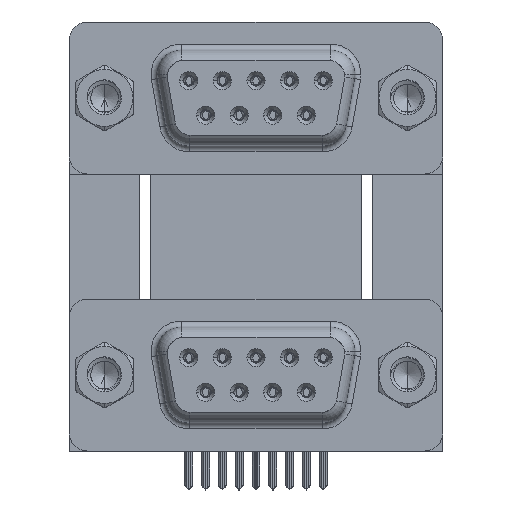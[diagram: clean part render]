
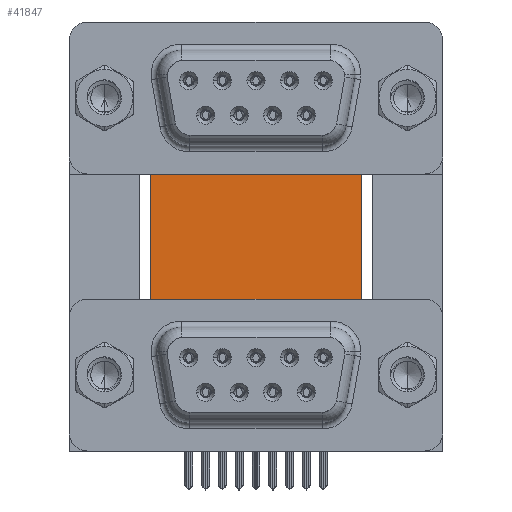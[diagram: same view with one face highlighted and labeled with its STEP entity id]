
A CAD part, top view. The second image highlights one B-rep face of the part: STEP entity #41847.
In plain terms, the highlighted planar face has unit normal (0, 0, 1).
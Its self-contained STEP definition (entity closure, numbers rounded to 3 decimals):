
#143 = EDGE_CURVE ( 'NONE', #31300, #3203, #23245, .T. ) ;
#572 = LINE ( 'NONE', #11947, #24037 ) ;
#943 = DIRECTION ( 'NONE',  ( -0.336, -0.942, 0. ) ) ;
#944 = LINE ( 'NONE', #15397, #3514 ) ;
#1466 = EDGE_CURVE ( 'NONE', #10846, #35164, #11918, .T. ) ;
#1846 = CARTESIAN_POINT ( 'NONE',  ( 3.79, 16.585, -12. ) ) ;
#2363 = VERTEX_POINT ( 'NONE', #5298 ) ;
#2872 = DIRECTION ( 'NONE',  ( 0., -1., 0. ) ) ;
#3203 = VERTEX_POINT ( 'NONE', #42561 ) ;
#3514 = VECTOR ( 'NONE', #33611, 1000. ) ;
#5298 = CARTESIAN_POINT ( 'NONE',  ( 3.79, 16.585, -12. ) ) ;
#5550 = LINE ( 'NONE', #23525, #19580 ) ;
#5804 = EDGE_CURVE ( 'NONE', #2363, #32591, #39345, .T. ) ;
#5820 = CARTESIAN_POINT ( 'NONE',  ( 22.59, -4.635, -12. ) ) ;
#6015 = EDGE_CURVE ( 'NONE', #22601, #10846, #944, .T. ) ;
#6263 = CARTESIAN_POINT ( 'NONE',  ( 2.9, -3.735, -12. ) ) ;
#6420 = ORIENTED_EDGE ( 'NONE', *, *, #22194, .T. ) ;
#8734 = FACE_OUTER_BOUND ( 'NONE', #43649, .T. ) ;
#10047 = VECTOR ( 'NONE', #26357, 1000. ) ;
#10072 = LINE ( 'NONE', #45401, #39113 ) ;
#10383 = DIRECTION ( 'NONE',  ( -0.336, 0.942, 0. ) ) ;
#10444 = VERTEX_POINT ( 'NONE', #33880 ) ;
#10846 = VERTEX_POINT ( 'NONE', #30279 ) ;
#11463 = LINE ( 'NONE', #18355, #26420 ) ;
#11918 = LINE ( 'NONE', #21882, #10047 ) ;
#11947 = CARTESIAN_POINT ( 'NONE',  ( 22.59, -4.635, -12. ) ) ;
#12884 = ORIENTED_EDGE ( 'NONE', *, *, #24307, .T. ) ;
#13352 = VERTEX_POINT ( 'NONE', #44751 ) ;
#13515 = VECTOR ( 'NONE', #943, 1000. ) ;
#13616 = EDGE_CURVE ( 'NONE', #2363, #31300, #21714, .T. ) ;
#13801 = VECTOR ( 'NONE', #21245, 1000. ) ;
#13911 = VERTEX_POINT ( 'NONE', #5820 ) ;
#13927 = ORIENTED_EDGE ( 'NONE', *, *, #6015, .T. ) ;
#15397 = CARTESIAN_POINT ( 'NONE',  ( 3.79, -3.735, -12. ) ) ;
#16994 = ORIENTED_EDGE ( 'NONE', *, *, #41532, .T. ) ;
#17718 = ORIENTED_EDGE ( 'NONE', *, *, #1466, .T. ) ;
#18168 = CARTESIAN_POINT ( 'NONE',  ( 21.2, 16.585, -12. ) ) ;
#18355 = CARTESIAN_POINT ( 'NONE',  ( 22.09, -4.635, -12. ) ) ;
#18534 = DIRECTION ( 'NONE',  ( 0., 0., -1. ) ) ;
#18956 = CARTESIAN_POINT ( 'NONE',  ( 2.4, -4.635, -12. ) ) ;
#19362 = ORIENTED_EDGE ( 'NONE', *, *, #37364, .T. ) ;
#19580 = VECTOR ( 'NONE', #20441, 1000. ) ;
#20441 = DIRECTION ( 'NONE',  ( 0., 1., 0. ) ) ;
#21245 = DIRECTION ( 'NONE',  ( 1., 0., 0. ) ) ;
#21714 = LINE ( 'NONE', #42338, #13801 ) ;
#21882 = CARTESIAN_POINT ( 'NONE',  ( 22.09, -3.735, -12. ) ) ;
#22131 = DIRECTION ( 'NONE',  ( 1., 0., 0. ) ) ;
#22194 = EDGE_CURVE ( 'NONE', #10444, #13352, #10072, .T. ) ;
#22601 = VERTEX_POINT ( 'NONE', #6263 ) ;
#23245 = LINE ( 'NONE', #30788, #34875 ) ;
#23525 = CARTESIAN_POINT ( 'NONE',  ( 2.9, -3.735, -12. ) ) ;
#24037 = VECTOR ( 'NONE', #10383, 1000. ) ;
#24307 = EDGE_CURVE ( 'NONE', #32591, #10444, #40762, .T. ) ;
#25619 = DIRECTION ( 'NONE',  ( -1., 0., 0. ) ) ;
#26357 = DIRECTION ( 'NONE',  ( 0., -1., 0. ) ) ;
#26420 = VECTOR ( 'NONE', #22131, 1000. ) ;
#26883 = ORIENTED_EDGE ( 'NONE', *, *, #13616, .F. ) ;
#27349 = DIRECTION ( 'NONE',  ( 1., 0., 0. ) ) ;
#28034 = ORIENTED_EDGE ( 'NONE', *, *, #5804, .T. ) ;
#28209 = EDGE_CURVE ( 'NONE', #35164, #13911, #11463, .T. ) ;
#28493 = VECTOR ( 'NONE', #2872, 1000. ) ;
#30279 = CARTESIAN_POINT ( 'NONE',  ( 22.09, -3.735, -12. ) ) ;
#30788 = CARTESIAN_POINT ( 'NONE',  ( 21.2, 16.585, -12. ) ) ;
#31300 = VERTEX_POINT ( 'NONE', #18168 ) ;
#32591 = VERTEX_POINT ( 'NONE', #43997 ) ;
#33449 = ORIENTED_EDGE ( 'NONE', *, *, #143, .F. ) ;
#33611 = DIRECTION ( 'NONE',  ( 1., 0., 0. ) ) ;
#33880 = CARTESIAN_POINT ( 'NONE',  ( 2.4, -4.635, -12. ) ) ;
#34048 = PLANE ( 'NONE',  #40825 ) ;
#34875 = VECTOR ( 'NONE', #37697, 1000. ) ;
#35164 = VERTEX_POINT ( 'NONE', #35418 ) ;
#35302 = CARTESIAN_POINT ( 'NONE',  ( 3.79, 16.585, -12. ) ) ;
#35418 = CARTESIAN_POINT ( 'NONE',  ( 22.09, -4.635, -12. ) ) ;
#37364 = EDGE_CURVE ( 'NONE', #13911, #3203, #572, .T. ) ;
#37697 = DIRECTION ( 'NONE',  ( 0., -1., 0. ) ) ;
#39113 = VECTOR ( 'NONE', #27349, 1000. ) ;
#39345 = LINE ( 'NONE', #35302, #28493 ) ;
#40762 = LINE ( 'NONE', #18956, #13515 ) ;
#40825 = AXIS2_PLACEMENT_3D ( 'NONE', #1846, #18534, #25619 ) ;
#41532 = EDGE_CURVE ( 'NONE', #13352, #22601, #5550, .T. ) ;
#41847 = ADVANCED_FACE ( 'NONE', ( #8734 ), #34048, .F. ) ;
#42194 = ORIENTED_EDGE ( 'NONE', *, *, #28209, .T. ) ;
#42338 = CARTESIAN_POINT ( 'NONE',  ( 3.79, 16.585, -12. ) ) ;
#42561 = CARTESIAN_POINT ( 'NONE',  ( 21.2, -0.735, -12. ) ) ;
#43649 = EDGE_LOOP ( 'NONE', ( #13927, #17718, #42194, #19362, #33449, #26883, #28034, #12884, #6420, #16994 ) ) ;
#43997 = CARTESIAN_POINT ( 'NONE',  ( 3.79, -0.735, -12. ) ) ;
#44751 = CARTESIAN_POINT ( 'NONE',  ( 2.9, -4.635, -12. ) ) ;
#45401 = CARTESIAN_POINT ( 'NONE',  ( 2.9, -4.635, -12. ) ) ;
